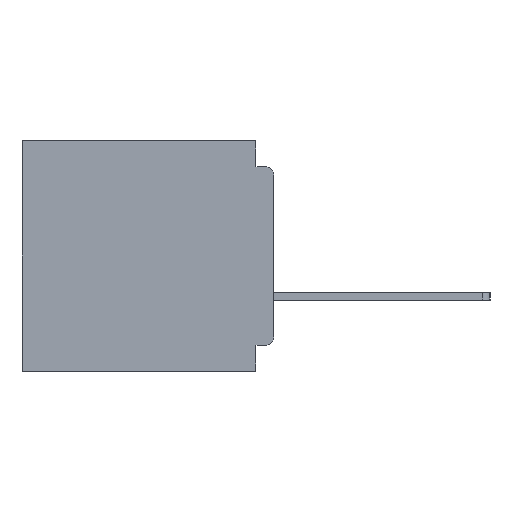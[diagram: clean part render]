
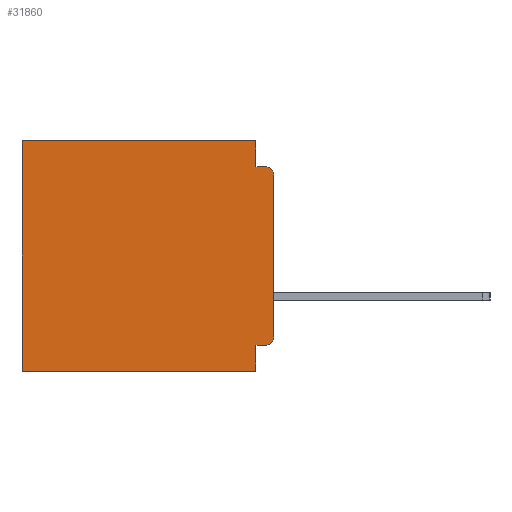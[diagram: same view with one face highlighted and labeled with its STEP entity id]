
A CAD part, left-side view. The second image highlights one B-rep face of the part: STEP entity #31860.
In plain terms, the highlighted planar face has unit normal (-1, 0, 0).
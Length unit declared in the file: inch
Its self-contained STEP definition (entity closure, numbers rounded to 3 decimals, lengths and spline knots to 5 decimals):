
#230 = EDGE_LOOP ( 'NONE', ( #24684, #2948, #11697, #17969, #18631, #10309, #38559, #9577, #35871, #5733 ) ) ;
#2076 = LINE ( 'NONE', #18966, #10779 ) ;
#2519 = VERTEX_POINT ( 'NONE', #15598 ) ;
#2932 = VERTEX_POINT ( 'NONE', #20471 ) ;
#2948 = ORIENTED_EDGE ( 'NONE', *, *, #5067, .T. ) ;
#4081 = FACE_OUTER_BOUND ( 'NONE', #230, .T. ) ;
#4131 = EDGE_CURVE ( 'NONE', #30894, #10683, #9469, .T. ) ;
#4925 = AXIS2_PLACEMENT_3D ( 'NONE', #26541, #7122, #29772 ) ;
#4996 = CARTESIAN_POINT ( 'NONE',  ( 0.3, 0., -0.34 ) ) ;
#5067 = EDGE_CURVE ( 'NONE', #28988, #2519, #29395, .T. ) ;
#5733 = ORIENTED_EDGE ( 'NONE', *, *, #41051, .T. ) ;
#5949 = VERTEX_POINT ( 'NONE', #21566 ) ;
#7122 = DIRECTION ( 'NONE',  ( -1., 0., 0. ) ) ;
#7155 = VERTEX_POINT ( 'NONE', #27507 ) ;
#7238 = VECTOR ( 'NONE', #40687, 39.37008 ) ;
#7548 = VECTOR ( 'NONE', #9655, 39.37008 ) ;
#7661 = DIRECTION ( 'NONE',  ( 0., 0., -1. ) ) ;
#9469 = LINE ( 'NONE', #19273, #34240 ) ;
#9577 = ORIENTED_EDGE ( 'NONE', *, *, #27408, .F. ) ;
#9585 = LINE ( 'NONE', #25853, #7548 ) ;
#9655 = DIRECTION ( 'NONE',  ( 0., 1., 0. ) ) ;
#10309 = ORIENTED_EDGE ( 'NONE', *, *, #4131, .T. ) ;
#10683 = VERTEX_POINT ( 'NONE', #22086 ) ;
#10760 = CARTESIAN_POINT ( 'NONE',  ( 0.3, 0., -0.06 ) ) ;
#10779 = VECTOR ( 'NONE', #35028, 39.37008 ) ;
#11697 = ORIENTED_EDGE ( 'NONE', *, *, #26474, .F. ) ;
#14021 = DIRECTION ( 'NONE',  ( -1., 0., 0. ) ) ;
#15598 = CARTESIAN_POINT ( 'NONE',  ( 0.3, 0.015, -0.045 ) ) ;
#16351 = DIRECTION ( 'NONE',  ( 0., 0., -1. ) ) ;
#17007 = VECTOR ( 'NONE', #40958, 39.37008 ) ;
#17119 = LINE ( 'NONE', #31313, #40708 ) ;
#17290 = CARTESIAN_POINT ( 'NONE',  ( 0.3, 0.031, -0.4 ) ) ;
#17969 = ORIENTED_EDGE ( 'NONE', *, *, #35432, .F. ) ;
#17998 = LINE ( 'NONE', #37763, #17007 ) ;
#18631 = ORIENTED_EDGE ( 'NONE', *, *, #25232, .T. ) ;
#18966 = CARTESIAN_POINT ( 'NONE',  ( 0.3, 0.031, -0.4 ) ) ;
#19251 = VECTOR ( 'NONE', #22310, 39.37008 ) ;
#19273 = CARTESIAN_POINT ( 'NONE',  ( 0.3, 0.437, -0.4 ) ) ;
#20471 = CARTESIAN_POINT ( 'NONE',  ( 0.3, 0.031, 0. ) ) ;
#20927 = DIRECTION ( 'NONE',  ( 0., 0., -1. ) ) ;
#21227 = EDGE_CURVE ( 'NONE', #28988, #30720, #27816, .T. ) ;
#21314 = EDGE_CURVE ( 'NONE', #5949, #24392, #9585, .T. ) ;
#21566 = CARTESIAN_POINT ( 'NONE',  ( 0.3, 0.015, -0.355 ) ) ;
#22086 = CARTESIAN_POINT ( 'NONE',  ( 0.3, 0.437, -0.4 ) ) ;
#22310 = DIRECTION ( 'NONE',  ( 0., 0., -1. ) ) ;
#23717 = CARTESIAN_POINT ( 'NONE',  ( 0.3, 0., -0.4 ) ) ;
#23865 = PLANE ( 'NONE',  #34549 ) ;
#24392 = VERTEX_POINT ( 'NONE', #27464 ) ;
#24448 = CIRCLE ( 'NONE', #41186, 0.015 ) ;
#24684 = ORIENTED_EDGE ( 'NONE', *, *, #21227, .F. ) ;
#25232 = EDGE_CURVE ( 'NONE', #2932, #30894, #17119, .T. ) ;
#25853 = CARTESIAN_POINT ( 'NONE',  ( 0.3, 0., -0.355 ) ) ;
#26474 = EDGE_CURVE ( 'NONE', #7155, #2519, #17998, .T. ) ;
#26541 = CARTESIAN_POINT ( 'NONE',  ( 0.3, 0.015, -0.06 ) ) ;
#27059 = DIRECTION ( 'NONE',  ( 1., 0., 0. ) ) ;
#27408 = EDGE_CURVE ( 'NONE', #24392, #35342, #2076, .T. ) ;
#27464 = CARTESIAN_POINT ( 'NONE',  ( 0.3, 0.031, -0.355 ) ) ;
#27507 = CARTESIAN_POINT ( 'NONE',  ( 0.3, 0.031, -0.045 ) ) ;
#27816 = LINE ( 'NONE', #41504, #19251 ) ;
#28168 = DIRECTION ( 'NONE',  ( 0., 1., 0. ) ) ;
#28988 = VERTEX_POINT ( 'NONE', #10760 ) ;
#29395 = CIRCLE ( 'NONE', #4925, 0.015 ) ;
#29772 = DIRECTION ( 'NONE',  ( 0., 0., -1. ) ) ;
#30653 = CARTESIAN_POINT ( 'NONE',  ( 0.3, 0.031, 0. ) ) ;
#30720 = VERTEX_POINT ( 'NONE', #4996 ) ;
#30894 = VERTEX_POINT ( 'NONE', #35169 ) ;
#31313 = CARTESIAN_POINT ( 'NONE',  ( 0.3, 0., 0. ) ) ;
#31356 = EDGE_CURVE ( 'NONE', #35342, #10683, #32080, .T. ) ;
#31860 = ADVANCED_FACE ( 'NONE', ( #4081 ), #23865, .F. ) ;
#32080 = LINE ( 'NONE', #37506, #7238 ) ;
#32609 = LINE ( 'NONE', #30653, #41059 ) ;
#33363 = CARTESIAN_POINT ( 'NONE',  ( 0.3, 0.015, -0.34 ) ) ;
#34240 = VECTOR ( 'NONE', #16351, 39.37008 ) ;
#34549 = AXIS2_PLACEMENT_3D ( 'NONE', #23717, #27059, #7661 ) ;
#35028 = DIRECTION ( 'NONE',  ( 0., 0., -1. ) ) ;
#35169 = CARTESIAN_POINT ( 'NONE',  ( 0.3, 0.437, 0. ) ) ;
#35342 = VERTEX_POINT ( 'NONE', #17290 ) ;
#35432 = EDGE_CURVE ( 'NONE', #2932, #7155, #32609, .T. ) ;
#35871 = ORIENTED_EDGE ( 'NONE', *, *, #21314, .F. ) ;
#36573 = DIRECTION ( 'NONE',  ( 0., 0., -1. ) ) ;
#37506 = CARTESIAN_POINT ( 'NONE',  ( 0.3, 0., -0.4 ) ) ;
#37763 = CARTESIAN_POINT ( 'NONE',  ( 0.3, 0., -0.045 ) ) ;
#38559 = ORIENTED_EDGE ( 'NONE', *, *, #31356, .F. ) ;
#40687 = DIRECTION ( 'NONE',  ( 0., 1., 0. ) ) ;
#40708 = VECTOR ( 'NONE', #28168, 39.37008 ) ;
#40958 = DIRECTION ( 'NONE',  ( 0., -1., 0. ) ) ;
#41051 = EDGE_CURVE ( 'NONE', #5949, #30720, #24448, .T. ) ;
#41059 = VECTOR ( 'NONE', #20927, 39.37008 ) ;
#41186 = AXIS2_PLACEMENT_3D ( 'NONE', #33363, #14021, #36573 ) ;
#41504 = CARTESIAN_POINT ( 'NONE',  ( 0.3, 0., -0.4 ) ) ;
